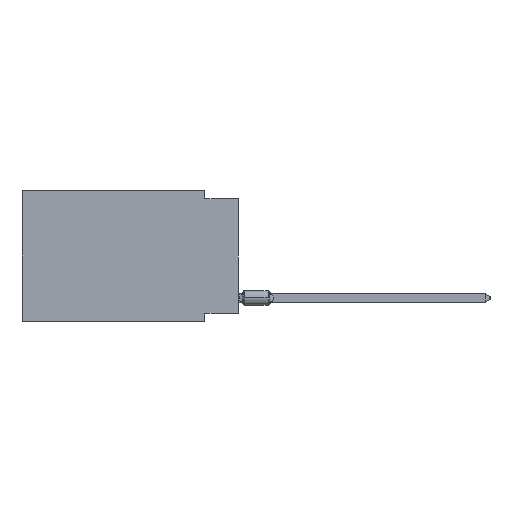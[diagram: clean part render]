
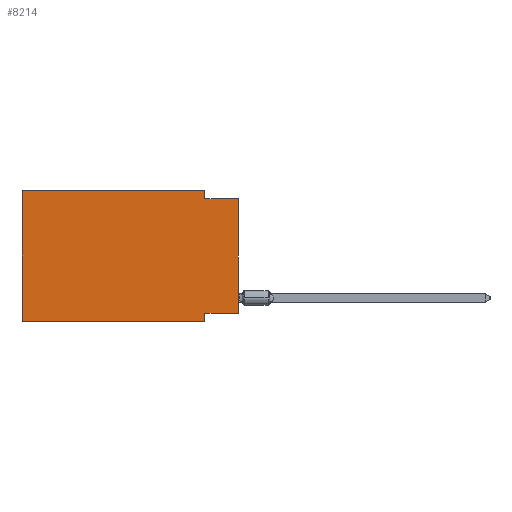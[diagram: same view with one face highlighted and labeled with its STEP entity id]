
A CAD part, left-side view. The second image highlights one B-rep face of the part: STEP entity #8214.
In plain terms, the highlighted planar face has unit normal (-1, 0, 0).
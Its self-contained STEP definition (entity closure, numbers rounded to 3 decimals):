
#1149 = EDGE_CURVE ( 'NONE', #50501, #17852, #29912, .T. ) ;
#2135 = LINE ( 'NONE', #33693, #32590 ) ;
#2359 = CARTESIAN_POINT ( 'NONE',  ( 0., 0., -0.635 ) ) ;
#5789 = DIRECTION ( 'NONE',  ( 1., 0., 0. ) ) ;
#6286 = DIRECTION ( 'NONE',  ( 0., 0., 1. ) ) ;
#6878 = VECTOR ( 'NONE', #15727, 1000. ) ;
#8214 = ADVANCED_FACE ( 'NONE', ( #13783 ), #49485, .F. ) ;
#8857 = DIRECTION ( 'NONE',  ( 0., 1., 0. ) ) ;
#9415 = CARTESIAN_POINT ( 'NONE',  ( 0., 16.383, 0. ) ) ;
#9712 = VECTOR ( 'NONE', #18012, 1000. ) ;
#10155 = LINE ( 'NONE', #30072, #32049 ) ;
#12100 = VERTEX_POINT ( 'NONE', #27714 ) ;
#12437 = EDGE_LOOP ( 'NONE', ( #47988, #21067, #31002, #42283, #32772, #48575, #47467, #17853 ) ) ;
#12734 = LINE ( 'NONE', #28519, #17108 ) ;
#13255 = CARTESIAN_POINT ( 'NONE',  ( 0., 0., -9.271 ) ) ;
#13356 = EDGE_CURVE ( 'NONE', #30188, #49411, #51110, .T. ) ;
#13783 = FACE_OUTER_BOUND ( 'NONE', #12437, .T. ) ;
#14009 = DIRECTION ( 'NONE',  ( 0., 0., -1. ) ) ;
#14358 = DIRECTION ( 'NONE',  ( 0., 0., -1. ) ) ;
#15727 = DIRECTION ( 'NONE',  ( 0., -1., 0. ) ) ;
#17108 = VECTOR ( 'NONE', #8857, 1000. ) ;
#17811 = DIRECTION ( 'NONE',  ( 0., 0., 1. ) ) ;
#17852 = VERTEX_POINT ( 'NONE', #19602 ) ;
#17853 = ORIENTED_EDGE ( 'NONE', *, *, #32438, .F. ) ;
#18012 = DIRECTION ( 'NONE',  ( 0., -1., 0. ) ) ;
#19382 = CARTESIAN_POINT ( 'NONE',  ( 0., 16.383, -9.906 ) ) ;
#19587 = VERTEX_POINT ( 'NONE', #19986 ) ;
#19602 = CARTESIAN_POINT ( 'NONE',  ( 0., 2.54, 0. ) ) ;
#19986 = CARTESIAN_POINT ( 'NONE',  ( 0., 2.54, -9.271 ) ) ;
#21067 = ORIENTED_EDGE ( 'NONE', *, *, #13356, .F. ) ;
#21474 = EDGE_CURVE ( 'NONE', #12100, #50501, #49879, .T. ) ;
#21888 = CARTESIAN_POINT ( 'NONE',  ( 0., 16.383, 0. ) ) ;
#22368 = VERTEX_POINT ( 'NONE', #34764 ) ;
#22901 = VECTOR ( 'NONE', #47998, 1000. ) ;
#23318 = VERTEX_POINT ( 'NONE', #13255 ) ;
#25197 = DIRECTION ( 'NONE',  ( 0., 0., -1. ) ) ;
#27714 = CARTESIAN_POINT ( 'NONE',  ( 0., 16.383, -9.906 ) ) ;
#28323 = CARTESIAN_POINT ( 'NONE',  ( 0., 16.383, 0. ) ) ;
#28519 = CARTESIAN_POINT ( 'NONE',  ( 0., 0., -9.271 ) ) ;
#29400 = EDGE_CURVE ( 'NONE', #19587, #22368, #2135, .T. ) ;
#29452 = CARTESIAN_POINT ( 'NONE',  ( 0., 16.383, 0. ) ) ;
#29912 = LINE ( 'NONE', #21888, #9712 ) ;
#30072 = CARTESIAN_POINT ( 'NONE',  ( 0., 0., 0. ) ) ;
#30188 = VERTEX_POINT ( 'NONE', #46164 ) ;
#31002 = ORIENTED_EDGE ( 'NONE', *, *, #33428, .F. ) ;
#32049 = VECTOR ( 'NONE', #6286, 1000. ) ;
#32438 = EDGE_CURVE ( 'NONE', #23318, #19587, #12734, .T. ) ;
#32590 = VECTOR ( 'NONE', #14009, 1000. ) ;
#32772 = ORIENTED_EDGE ( 'NONE', *, *, #21474, .F. ) ;
#33428 = EDGE_CURVE ( 'NONE', #17852, #30188, #49788, .T. ) ;
#33693 = CARTESIAN_POINT ( 'NONE',  ( 0., 2.54, -9.906 ) ) ;
#33800 = EDGE_CURVE ( 'NONE', #23318, #49411, #10155, .T. ) ;
#34764 = CARTESIAN_POINT ( 'NONE',  ( 0., 2.54, -9.906 ) ) ;
#37238 = EDGE_CURVE ( 'NONE', #12100, #22368, #51164, .T. ) ;
#38945 = AXIS2_PLACEMENT_3D ( 'NONE', #9415, #5789, #25197 ) ;
#40227 = VECTOR ( 'NONE', #17811, 1000. ) ;
#42009 = VECTOR ( 'NONE', #14358, 1000. ) ;
#42283 = ORIENTED_EDGE ( 'NONE', *, *, #1149, .F. ) ;
#46164 = CARTESIAN_POINT ( 'NONE',  ( 0., 2.54, -0.635 ) ) ;
#47467 = ORIENTED_EDGE ( 'NONE', *, *, #29400, .F. ) ;
#47736 = CARTESIAN_POINT ( 'NONE',  ( 0., 0., -0.635 ) ) ;
#47988 = ORIENTED_EDGE ( 'NONE', *, *, #33800, .T. ) ;
#47998 = DIRECTION ( 'NONE',  ( 0., -1., 0. ) ) ;
#48575 = ORIENTED_EDGE ( 'NONE', *, *, #37238, .T. ) ;
#49411 = VERTEX_POINT ( 'NONE', #2359 ) ;
#49485 = PLANE ( 'NONE',  #38945 ) ;
#49788 = LINE ( 'NONE', #50037, #42009 ) ;
#49879 = LINE ( 'NONE', #29452, #40227 ) ;
#50037 = CARTESIAN_POINT ( 'NONE',  ( 0., 2.54, 0. ) ) ;
#50501 = VERTEX_POINT ( 'NONE', #28323 ) ;
#51110 = LINE ( 'NONE', #47736, #22901 ) ;
#51164 = LINE ( 'NONE', #19382, #6878 ) ;
